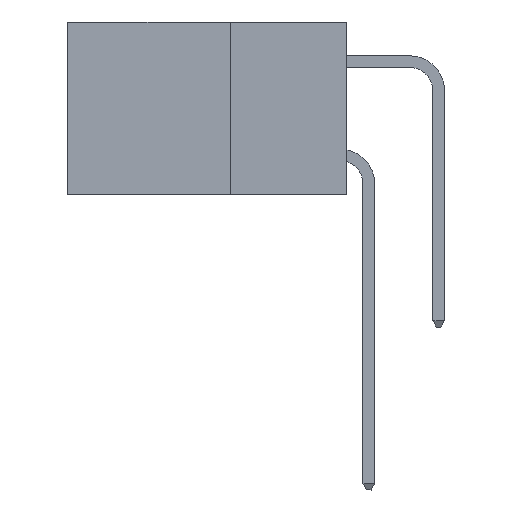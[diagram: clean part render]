
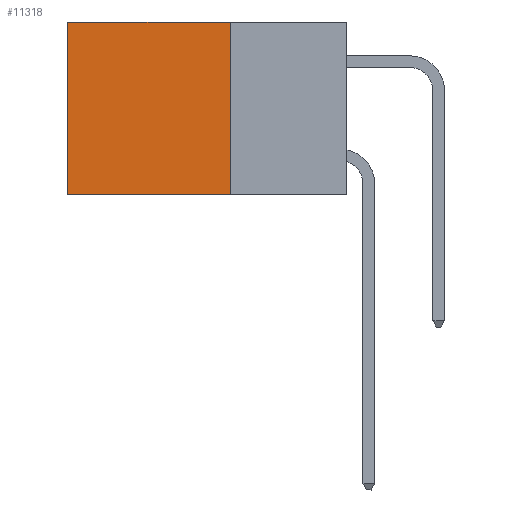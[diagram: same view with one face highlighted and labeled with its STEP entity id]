
A CAD part, left-side view. The second image highlights one B-rep face of the part: STEP entity #11318.
In plain terms, the highlighted planar face has unit normal (-1, 0, 0).
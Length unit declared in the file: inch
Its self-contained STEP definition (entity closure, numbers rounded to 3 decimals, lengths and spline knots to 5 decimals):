
#101 = EDGE_CURVE ( 'NONE', #8702, #10225, #9782, .T. ) ;
#764 = CARTESIAN_POINT ( 'NONE',  ( 0.2875, 0.25, 0. ) ) ;
#865 = DIRECTION ( 'NONE',  ( 0., 1., 0. ) ) ;
#1107 = CARTESIAN_POINT ( 'NONE',  ( 0.2875, 0.25, 0. ) ) ;
#1850 = FACE_OUTER_BOUND ( 'NONE', #8752, .T. ) ;
#2185 = CARTESIAN_POINT ( 'NONE',  ( 0.2875, 0.25, 0. ) ) ;
#3226 = VECTOR ( 'NONE', #11018, 39.37008 ) ;
#3380 = EDGE_CURVE ( 'NONE', #6150, #7802, #8732, .T. ) ;
#3541 = ORIENTED_EDGE ( 'NONE', *, *, #3380, .F. ) ;
#3839 = CARTESIAN_POINT ( 'NONE',  ( 0.2875, 0.25, -0.37 ) ) ;
#4338 = CARTESIAN_POINT ( 'NONE',  ( 0.2875, 0.6, 0. ) ) ;
#5197 = VECTOR ( 'NONE', #8017, 39.37008 ) ;
#5294 = VECTOR ( 'NONE', #865, 39.37008 ) ;
#5792 = CARTESIAN_POINT ( 'NONE',  ( 0.2875, 0.6, -0.37 ) ) ;
#6150 = VERTEX_POINT ( 'NONE', #1107 ) ;
#6257 = VECTOR ( 'NONE', #13208, 39.37008 ) ;
#6584 = DIRECTION ( 'NONE',  ( 0., 0., -1. ) ) ;
#6617 = CARTESIAN_POINT ( 'NONE',  ( 0.2875, 0.6, 0. ) ) ;
#7650 = EDGE_CURVE ( 'NONE', #7802, #10225, #11741, .T. ) ;
#7802 = VERTEX_POINT ( 'NONE', #9857 ) ;
#7872 = LINE ( 'NONE', #10236, #5197 ) ;
#8017 = DIRECTION ( 'NONE',  ( 0., 1., 0. ) ) ;
#8702 = VERTEX_POINT ( 'NONE', #4338 ) ;
#8732 = LINE ( 'NONE', #2185, #6257 ) ;
#8752 = EDGE_LOOP ( 'NONE', ( #9529, #11011, #3541, #9309 ) ) ;
#9309 = ORIENTED_EDGE ( 'NONE', *, *, #11720, .T. ) ;
#9529 = ORIENTED_EDGE ( 'NONE', *, *, #101, .T. ) ;
#9782 = LINE ( 'NONE', #6617, #3226 ) ;
#9857 = CARTESIAN_POINT ( 'NONE',  ( 0.2875, 0.25, -0.37 ) ) ;
#10027 = AXIS2_PLACEMENT_3D ( 'NONE', #764, #10913, #6584 ) ;
#10225 = VERTEX_POINT ( 'NONE', #5792 ) ;
#10236 = CARTESIAN_POINT ( 'NONE',  ( 0.2875, 0.25, 0. ) ) ;
#10623 = PLANE ( 'NONE',  #10027 ) ;
#10913 = DIRECTION ( 'NONE',  ( 1., 0., 0. ) ) ;
#11011 = ORIENTED_EDGE ( 'NONE', *, *, #7650, .F. ) ;
#11018 = DIRECTION ( 'NONE',  ( 0., 0., -1. ) ) ;
#11318 = ADVANCED_FACE ( 'NONE', ( #1850 ), #10623, .F. ) ;
#11720 = EDGE_CURVE ( 'NONE', #6150, #8702, #7872, .T. ) ;
#11741 = LINE ( 'NONE', #3839, #5294 ) ;
#13208 = DIRECTION ( 'NONE',  ( 0., 0., -1. ) ) ;
